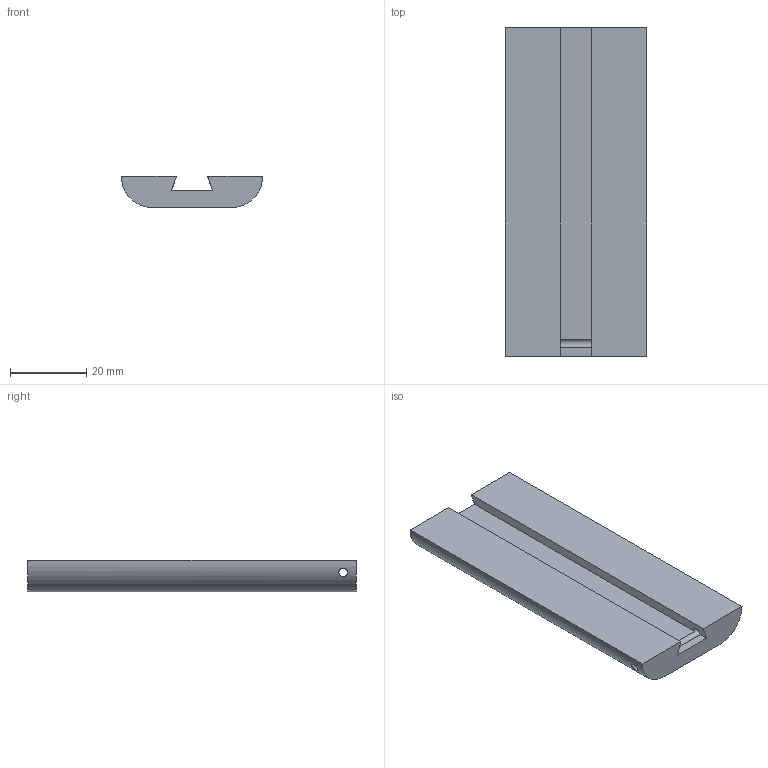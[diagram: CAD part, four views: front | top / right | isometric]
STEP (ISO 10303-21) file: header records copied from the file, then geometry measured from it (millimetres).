
FILE_DESCRIPTION(/* description */ (''),/* implementation_level */ '2;1');
FILE_NAME(/* name */ 'Base Slip Cover v1.step',/* time_stamp */ '2020-06-28T23:16:43-04:00',/* author */ (''),/* organization */ (''),/* preprocessor_version */ 'ST-DEVELOPER v18.1',/* originating_system */ 'Autodesk Translation Framework v9.3.0.1241',/* authorisation */ '');
FILE_SCHEMA (('AUTOMOTIVE_DESIGN { 1 0 10303 214 3 1 1 }'));
Length unit declared in the file: millimetre
Products named in the file (1): Base Slip Cover
Bounding box: 37 x 86 x 8.15 mm (x, y, z)
Volume: 20381.5 mm3; surface area: 8696.8 mm2
Topology: 1 solids, 1 shells, 12 faces, 38 edges, 26 vertices
Faces by surface type: plane 9, cylinder 3
Full cylindrical faces by diameter (mm): 2.25 x1
Entity records: 527 total; most frequent: CARTESIAN_POINT 145, ORIENTED_EDGE 76, DIRECTION 68, EDGE_CURVE 38, LINE 26, VECTOR 26, VERTEX_POINT 26, AXIS2_PLACEMENT_3D 21
